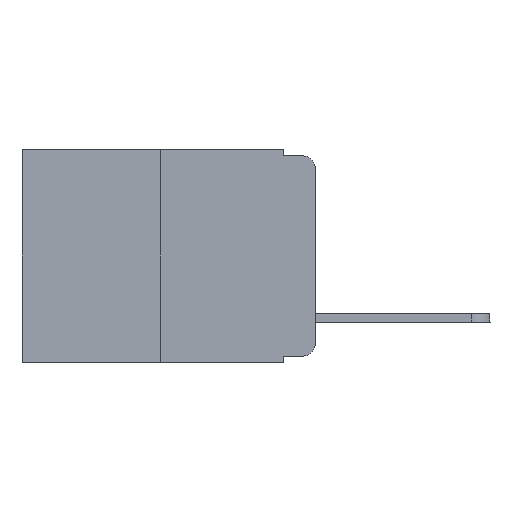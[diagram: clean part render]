
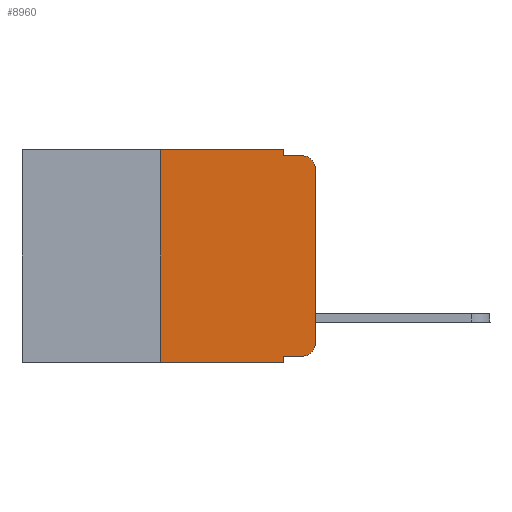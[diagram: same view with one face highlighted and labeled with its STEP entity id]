
A CAD part, left-side view. The second image highlights one B-rep face of the part: STEP entity #8960.
In plain terms, the highlighted planar face has unit normal (-1, 0, 0).
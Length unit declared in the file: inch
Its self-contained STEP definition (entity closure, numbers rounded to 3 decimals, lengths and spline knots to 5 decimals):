
#364 = DIRECTION ( 'NONE',  ( 0., 0., 1. ) ) ;
#698 = DIRECTION ( 'NONE',  ( 1., 0., 0. ) ) ;
#911 = VERTEX_POINT ( 'NONE', #23209 ) ;
#964 = EDGE_CURVE ( 'NONE', #23242, #6344, #17786, .T. ) ;
#1313 = DIRECTION ( 'NONE',  ( -1., 0., 0. ) ) ;
#1658 = CARTESIAN_POINT ( 'NONE',  ( 0., 0.02, -0.03 ) ) ;
#1878 = EDGE_CURVE ( 'NONE', #9953, #7697, #24188, .T. ) ;
#2048 = DIRECTION ( 'NONE',  ( -1., 0., 0. ) ) ;
#2205 = DIRECTION ( 'NONE',  ( 0., 0., -1. ) ) ;
#2527 = CARTESIAN_POINT ( 'NONE',  ( 0., 0.051, -0.01 ) ) ;
#3871 = ORIENTED_EDGE ( 'NONE', *, *, #22333, .F. ) ;
#3930 = DIRECTION ( 'NONE',  ( 0., 0., -1. ) ) ;
#4100 = EDGE_CURVE ( 'NONE', #21562, #6344, #7454, .T. ) ;
#4591 = LINE ( 'NONE', #10326, #12556 ) ;
#4679 = CARTESIAN_POINT ( 'NONE',  ( 0., 0.051, 0. ) ) ;
#5132 = LINE ( 'NONE', #13029, #6025 ) ;
#5451 = EDGE_CURVE ( 'NONE', #15040, #24505, #18445, .T. ) ;
#5560 = EDGE_CURVE ( 'NONE', #24505, #19253, #4591, .T. ) ;
#5575 = EDGE_CURVE ( 'NONE', #21562, #11422, #15653, .T. ) ;
#6025 = VECTOR ( 'NONE', #18968, 39.37008 ) ;
#6344 = VERTEX_POINT ( 'NONE', #17023 ) ;
#6730 = AXIS2_PLACEMENT_3D ( 'NONE', #19990, #698, #21944 ) ;
#6848 = LINE ( 'NONE', #4679, #13589 ) ;
#7353 = ORIENTED_EDGE ( 'NONE', *, *, #5451, .T. ) ;
#7454 = LINE ( 'NONE', #8760, #20622 ) ;
#7579 = EDGE_CURVE ( 'NONE', #19253, #7697, #25065, .T. ) ;
#7695 = ORIENTED_EDGE ( 'NONE', *, *, #5560, .T. ) ;
#7697 = VERTEX_POINT ( 'NONE', #20274 ) ;
#7873 = ORIENTED_EDGE ( 'NONE', *, *, #4100, .T. ) ;
#8173 = CARTESIAN_POINT ( 'NONE',  ( 0., 0., -0.03 ) ) ;
#8374 = ORIENTED_EDGE ( 'NONE', *, *, #5575, .F. ) ;
#8760 = CARTESIAN_POINT ( 'NONE',  ( 0., 0.473, -0.343 ) ) ;
#8854 = DIRECTION ( 'NONE',  ( 0., -1., 0. ) ) ;
#8960 = ADVANCED_FACE ( 'NONE', ( #14209 ), #12164, .F. ) ;
#9206 = VECTOR ( 'NONE', #3930, 39.37008 ) ;
#9283 = EDGE_CURVE ( 'NONE', #911, #9953, #6848, .T. ) ;
#9689 = CARTESIAN_POINT ( 'NONE',  ( 0., 0.25, -0.343 ) ) ;
#9853 = CARTESIAN_POINT ( 'NONE',  ( 0., 0.02, -0.333 ) ) ;
#9922 = CARTESIAN_POINT ( 'NONE',  ( 0., 0.02, -0.313 ) ) ;
#9953 = VERTEX_POINT ( 'NONE', #12877 ) ;
#10326 = CARTESIAN_POINT ( 'NONE',  ( 0., 0., 0. ) ) ;
#10711 = ORIENTED_EDGE ( 'NONE', *, *, #10908, .T. ) ;
#10908 = EDGE_CURVE ( 'NONE', #23242, #15040, #14995, .T. ) ;
#11422 = VERTEX_POINT ( 'NONE', #15964 ) ;
#12164 = PLANE ( 'NONE',  #6730 ) ;
#12501 = CARTESIAN_POINT ( 'NONE',  ( 0., 0., -0.313 ) ) ;
#12556 = VECTOR ( 'NONE', #364, 39.37008 ) ;
#12877 = CARTESIAN_POINT ( 'NONE',  ( 0., 0.051, -0.01 ) ) ;
#13029 = CARTESIAN_POINT ( 'NONE',  ( 0., 0.473, 0. ) ) ;
#13589 = VECTOR ( 'NONE', #14453, 39.37008 ) ;
#14209 = FACE_OUTER_BOUND ( 'NONE', #21015, .T. ) ;
#14453 = DIRECTION ( 'NONE',  ( 0., 0., -1. ) ) ;
#14995 = LINE ( 'NONE', #24387, #16858 ) ;
#15040 = VERTEX_POINT ( 'NONE', #9853 ) ;
#15334 = DIRECTION ( 'NONE',  ( 0., 0., -1. ) ) ;
#15653 = LINE ( 'NONE', #23965, #23646 ) ;
#15964 = CARTESIAN_POINT ( 'NONE',  ( 0., 0.25, 0. ) ) ;
#16216 = DIRECTION ( 'NONE',  ( 0., -1., 0. ) ) ;
#16858 = VECTOR ( 'NONE', #8854, 39.37008 ) ;
#17023 = CARTESIAN_POINT ( 'NONE',  ( 0., 0.051, -0.343 ) ) ;
#17786 = LINE ( 'NONE', #23427, #9206 ) ;
#18044 = AXIS2_PLACEMENT_3D ( 'NONE', #1658, #1313, #15334 ) ;
#18445 = CIRCLE ( 'NONE', #24238, 0.02 ) ;
#18542 = ORIENTED_EDGE ( 'NONE', *, *, #9283, .F. ) ;
#18633 = DIRECTION ( 'NONE',  ( 0., -1., 0. ) ) ;
#18968 = DIRECTION ( 'NONE',  ( 0., -1., 0. ) ) ;
#19253 = VERTEX_POINT ( 'NONE', #8173 ) ;
#19990 = CARTESIAN_POINT ( 'NONE',  ( 0., 0.473, 0. ) ) ;
#20166 = DIRECTION ( 'NONE',  ( 0., 0., 1. ) ) ;
#20274 = CARTESIAN_POINT ( 'NONE',  ( 0., 0.02, -0.01 ) ) ;
#20622 = VECTOR ( 'NONE', #18633, 39.37008 ) ;
#21015 = EDGE_LOOP ( 'NONE', ( #7695, #23175, #23121, #18542, #3871, #8374, #7873, #25145, #10711, #7353 ) ) ;
#21348 = CARTESIAN_POINT ( 'NONE',  ( 0., 0.051, -0.333 ) ) ;
#21562 = VERTEX_POINT ( 'NONE', #9689 ) ;
#21944 = DIRECTION ( 'NONE',  ( 0., 0., -1. ) ) ;
#22333 = EDGE_CURVE ( 'NONE', #11422, #911, #5132, .T. ) ;
#23121 = ORIENTED_EDGE ( 'NONE', *, *, #1878, .F. ) ;
#23175 = ORIENTED_EDGE ( 'NONE', *, *, #7579, .T. ) ;
#23209 = CARTESIAN_POINT ( 'NONE',  ( 0., 0.051, 0. ) ) ;
#23242 = VERTEX_POINT ( 'NONE', #21348 ) ;
#23427 = CARTESIAN_POINT ( 'NONE',  ( 0., 0.051, 0. ) ) ;
#23646 = VECTOR ( 'NONE', #20166, 39.37008 ) ;
#23965 = CARTESIAN_POINT ( 'NONE',  ( 0., 0.25, 0. ) ) ;
#24188 = LINE ( 'NONE', #2527, #24489 ) ;
#24238 = AXIS2_PLACEMENT_3D ( 'NONE', #9922, #2048, #2205 ) ;
#24387 = CARTESIAN_POINT ( 'NONE',  ( 0., 0.051, -0.333 ) ) ;
#24489 = VECTOR ( 'NONE', #16216, 39.37008 ) ;
#24505 = VERTEX_POINT ( 'NONE', #12501 ) ;
#25065 = CIRCLE ( 'NONE', #18044, 0.02 ) ;
#25145 = ORIENTED_EDGE ( 'NONE', *, *, #964, .F. ) ;
